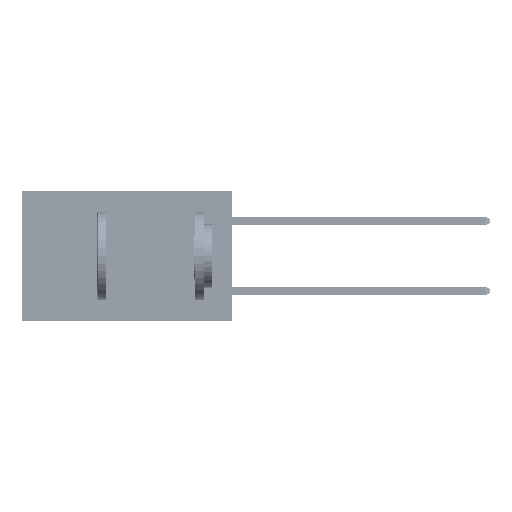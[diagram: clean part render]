
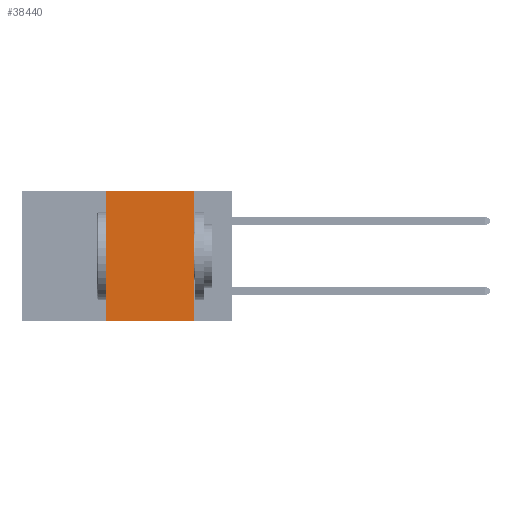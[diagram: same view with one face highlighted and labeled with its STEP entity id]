
A CAD part, left-side view. The second image highlights one B-rep face of the part: STEP entity #38440.
In plain terms, the highlighted planar face has unit normal (-1, 0, 0).
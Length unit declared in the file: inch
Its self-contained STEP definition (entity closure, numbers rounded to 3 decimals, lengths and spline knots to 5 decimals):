
#271 = EDGE_LOOP ( 'NONE', ( #19276, #9399, #25751, #4083 ) ) ;
#272 = DIRECTION ( 'NONE',  ( 0., 0., -1. ) ) ;
#932 = CARTESIAN_POINT ( 'NONE',  ( 0., 0.36, 0. ) ) ;
#1322 = EDGE_CURVE ( 'NONE', #39003, #3935, #26456, .T. ) ;
#3935 = VERTEX_POINT ( 'NONE', #932 ) ;
#4083 = ORIENTED_EDGE ( 'NONE', *, *, #45939, .T. ) ;
#7314 = EDGE_CURVE ( 'NONE', #3935, #8109, #11414, .T. ) ;
#8109 = VERTEX_POINT ( 'NONE', #17778 ) ;
#9399 = ORIENTED_EDGE ( 'NONE', *, *, #7314, .F. ) ;
#10486 = PLANE ( 'NONE',  #41192 ) ;
#10547 = CARTESIAN_POINT ( 'NONE',  ( 0., 0.6, -0.37 ) ) ;
#11414 = LINE ( 'NONE', #43227, #22918 ) ;
#12491 = DIRECTION ( 'NONE',  ( 0., -1., 0. ) ) ;
#14389 = VECTOR ( 'NONE', #20146, 39.37008 ) ;
#15299 = EDGE_CURVE ( 'NONE', #8109, #24163, #26829, .T. ) ;
#17422 = FACE_OUTER_BOUND ( 'NONE', #271, .T. ) ;
#17778 = CARTESIAN_POINT ( 'NONE',  ( 0., 0.11, 0. ) ) ;
#18463 = DIRECTION ( 'NONE',  ( 0., 0., -1. ) ) ;
#19276 = ORIENTED_EDGE ( 'NONE', *, *, #15299, .F. ) ;
#20146 = DIRECTION ( 'NONE',  ( 0., 0., 1. ) ) ;
#22918 = VECTOR ( 'NONE', #12491, 39.37008 ) ;
#24163 = VERTEX_POINT ( 'NONE', #24395 ) ;
#24395 = CARTESIAN_POINT ( 'NONE',  ( 0., 0.11, -0.37 ) ) ;
#25751 = ORIENTED_EDGE ( 'NONE', *, *, #1322, .F. ) ;
#26371 = VECTOR ( 'NONE', #37626, 39.37008 ) ;
#26456 = LINE ( 'NONE', #43257, #14389 ) ;
#26829 = LINE ( 'NONE', #42542, #28639 ) ;
#28639 = VECTOR ( 'NONE', #272, 39.37008 ) ;
#34181 = CARTESIAN_POINT ( 'NONE',  ( 0., 0.6, 0. ) ) ;
#36671 = LINE ( 'NONE', #10547, #26371 ) ;
#37626 = DIRECTION ( 'NONE',  ( 0., -1., 0. ) ) ;
#38440 = ADVANCED_FACE ( 'NONE', ( #17422 ), #10486, .F. ) ;
#39003 = VERTEX_POINT ( 'NONE', #48952 ) ;
#41192 = AXIS2_PLACEMENT_3D ( 'NONE', #34181, #41600, #18463 ) ;
#41600 = DIRECTION ( 'NONE',  ( 1., 0., 0. ) ) ;
#42542 = CARTESIAN_POINT ( 'NONE',  ( 0., 0.11, 0. ) ) ;
#43227 = CARTESIAN_POINT ( 'NONE',  ( 0., 0.6, 0. ) ) ;
#43257 = CARTESIAN_POINT ( 'NONE',  ( 0., 0.36, 0. ) ) ;
#45939 = EDGE_CURVE ( 'NONE', #39003, #24163, #36671, .T. ) ;
#48952 = CARTESIAN_POINT ( 'NONE',  ( 0., 0.36, -0.37 ) ) ;
